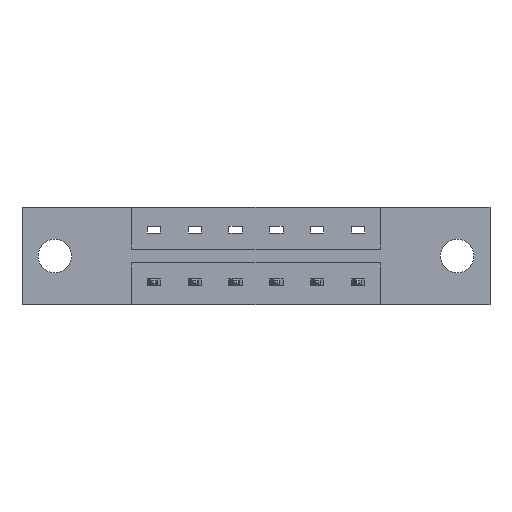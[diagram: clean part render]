
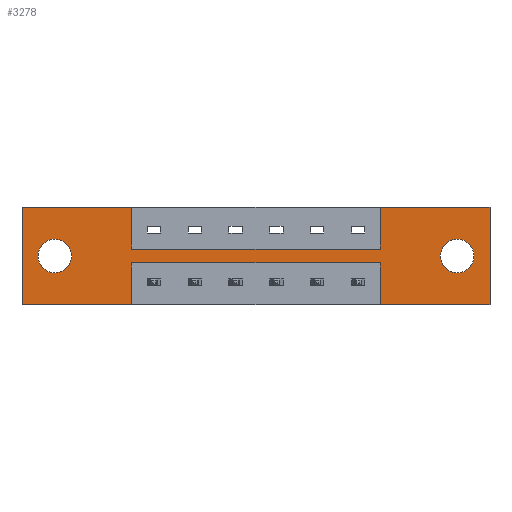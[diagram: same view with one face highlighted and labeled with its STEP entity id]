
A CAD part, front view. The second image highlights one B-rep face of the part: STEP entity #3278.
In plain terms, the highlighted planar face has unit normal (0, -1, 0).
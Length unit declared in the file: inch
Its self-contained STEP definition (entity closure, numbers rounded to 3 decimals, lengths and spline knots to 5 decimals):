
#50 = EDGE_CURVE ( 'NONE', #3558, #2212, #6643, .T. ) ;
#74 = CIRCLE ( 'NONE', #6820, 0.064 ) ;
#160 = DIRECTION ( 'NONE',  ( 0., 0., -1. ) ) ;
#168 = ORIENTED_EDGE ( 'NONE', *, *, #7767, .F. ) ;
#190 = CARTESIAN_POINT ( 'NONE',  ( 1.3665, 0., 0. ) ) ;
#343 = CARTESIAN_POINT ( 'NONE',  ( 1.784, 0., -0.37 ) ) ;
#434 = VECTOR ( 'NONE', #5804, 39.37008 ) ;
#483 = LINE ( 'NONE', #8229, #7252 ) ;
#489 = DIRECTION ( 'NONE',  ( -1., 0., 0. ) ) ;
#573 = LINE ( 'NONE', #5742, #3854 ) ;
#639 = VECTOR ( 'NONE', #5805, 39.37008 ) ;
#731 = ORIENTED_EDGE ( 'NONE', *, *, #4554, .F. ) ;
#736 = CIRCLE ( 'NONE', #7083, 0.064 ) ;
#845 = CARTESIAN_POINT ( 'NONE',  ( 0.4175, 0., -0.1585 ) ) ;
#866 = CARTESIAN_POINT ( 'NONE',  ( 0.125, 0., -0.185 ) ) ;
#899 = ORIENTED_EDGE ( 'NONE', *, *, #7003, .F. ) ;
#901 = ORIENTED_EDGE ( 'NONE', *, *, #7945, .F. ) ;
#948 = DIRECTION ( 'NONE',  ( 0., 0., -1. ) ) ;
#1079 = DIRECTION ( 'NONE',  ( -1., 0., 0. ) ) ;
#1104 = VERTEX_POINT ( 'NONE', #1747 ) ;
#1106 = CARTESIAN_POINT ( 'NONE',  ( 0., 0., -0.37 ) ) ;
#1258 = LINE ( 'NONE', #4473, #4813 ) ;
#1288 = ORIENTED_EDGE ( 'NONE', *, *, #2290, .F. ) ;
#1340 = VERTEX_POINT ( 'NONE', #7374 ) ;
#1341 = FACE_BOUND ( 'NONE', #5637, .T. ) ;
#1344 = VERTEX_POINT ( 'NONE', #4782 ) ;
#1371 = DIRECTION ( 'NONE',  ( 0., 1., 0. ) ) ;
#1386 = VERTEX_POINT ( 'NONE', #343 ) ;
#1469 = LINE ( 'NONE', #5368, #7797 ) ;
#1497 = LINE ( 'NONE', #4253, #4537 ) ;
#1504 = ORIENTED_EDGE ( 'NONE', *, *, #5845, .F. ) ;
#1539 = DIRECTION ( 'NONE',  ( 0., 0., -1. ) ) ;
#1661 = CARTESIAN_POINT ( 'NONE',  ( 1.3665, 0., -0.2115 ) ) ;
#1742 = DIRECTION ( 'NONE',  ( 0., 1., 0. ) ) ;
#1744 = ORIENTED_EDGE ( 'NONE', *, *, #50, .F. ) ;
#1747 = CARTESIAN_POINT ( 'NONE',  ( 1.659, 0., -0.121 ) ) ;
#1804 = CARTESIAN_POINT ( 'NONE',  ( 1.784, 0., 0. ) ) ;
#1864 = DIRECTION ( 'NONE',  ( -1., 0., 0. ) ) ;
#1870 = VERTEX_POINT ( 'NONE', #3134 ) ;
#1988 = VECTOR ( 'NONE', #3894, 39.37008 ) ;
#2088 = VECTOR ( 'NONE', #489, 39.37008 ) ;
#2092 = EDGE_CURVE ( 'NONE', #1340, #1344, #5871, .T. ) ;
#2192 = CARTESIAN_POINT ( 'NONE',  ( 1.659, 0., -0.249 ) ) ;
#2212 = VERTEX_POINT ( 'NONE', #6166 ) ;
#2283 = VERTEX_POINT ( 'NONE', #6288 ) ;
#2290 = EDGE_CURVE ( 'NONE', #6477, #2283, #4339, .T. ) ;
#2296 = EDGE_LOOP ( 'NONE', ( #901, #2449, #5321, #168, #4443, #1744, #6154, #899, #731, #1288, #1504, #3020 ) ) ;
#2305 = ORIENTED_EDGE ( 'NONE', *, *, #4058, .T. ) ;
#2449 = ORIENTED_EDGE ( 'NONE', *, *, #5718, .F. ) ;
#2600 = VERTEX_POINT ( 'NONE', #6654 ) ;
#2734 = ORIENTED_EDGE ( 'NONE', *, *, #2092, .T. ) ;
#2772 = VERTEX_POINT ( 'NONE', #6682 ) ;
#3020 = ORIENTED_EDGE ( 'NONE', *, *, #5200, .F. ) ;
#3050 = VECTOR ( 'NONE', #948, 39.37008 ) ;
#3134 = CARTESIAN_POINT ( 'NONE',  ( 1.3665, 0., -0.37 ) ) ;
#3217 = DIRECTION ( 'NONE',  ( 0., 0., 1. ) ) ;
#3278 = ADVANCED_FACE ( 'NONE', ( #5245, #1341, #7854 ), #3344, .T. ) ;
#3344 = PLANE ( 'NONE',  #5326 ) ;
#3387 = DIRECTION ( 'NONE',  ( 0., 1., 0. ) ) ;
#3558 = VERTEX_POINT ( 'NONE', #7043 ) ;
#3772 = DIRECTION ( 'NONE',  ( 1., 0., 0. ) ) ;
#3773 = LINE ( 'NONE', #1804, #1988 ) ;
#3792 = CARTESIAN_POINT ( 'NONE',  ( 0., 0., -0.37 ) ) ;
#3852 = AXIS2_PLACEMENT_3D ( 'NONE', #7090, #3387, #7850 ) ;
#3854 = VECTOR ( 'NONE', #3217, 39.37008 ) ;
#3860 = EDGE_CURVE ( 'NONE', #2772, #3558, #5482, .T. ) ;
#3894 = DIRECTION ( 'NONE',  ( 0., 0., -1. ) ) ;
#4058 = EDGE_CURVE ( 'NONE', #1104, #4666, #736, .T. ) ;
#4107 = ORIENTED_EDGE ( 'NONE', *, *, #7725, .T. ) ;
#4177 = CARTESIAN_POINT ( 'NONE',  ( 1.659, 0., -0.185 ) ) ;
#4253 = CARTESIAN_POINT ( 'NONE',  ( 0., 0., 0. ) ) ;
#4339 = LINE ( 'NONE', #3792, #2088 ) ;
#4369 = DIRECTION ( 'NONE',  ( 0., 0., -1. ) ) ;
#4417 = CARTESIAN_POINT ( 'NONE',  ( 0.4175, 0., -0.2115 ) ) ;
#4443 = ORIENTED_EDGE ( 'NONE', *, *, #6187, .F. ) ;
#4473 = CARTESIAN_POINT ( 'NONE',  ( 0., 0., 0. ) ) ;
#4492 = EDGE_CURVE ( 'NONE', #4607, #1386, #3773, .T. ) ;
#4537 = VECTOR ( 'NONE', #6830, 39.37008 ) ;
#4554 = EDGE_CURVE ( 'NONE', #2283, #6061, #1469, .T. ) ;
#4570 = CARTESIAN_POINT ( 'NONE',  ( 0.4175, 0., -0.2115 ) ) ;
#4607 = VERTEX_POINT ( 'NONE', #7315 ) ;
#4608 = LINE ( 'NONE', #4570, #639 ) ;
#4666 = VERTEX_POINT ( 'NONE', #2192 ) ;
#4782 = CARTESIAN_POINT ( 'NONE',  ( 0.125, 0., -0.121 ) ) ;
#4813 = VECTOR ( 'NONE', #3772, 39.37008 ) ;
#4914 = VERTEX_POINT ( 'NONE', #190 ) ;
#5200 = EDGE_CURVE ( 'NONE', #7674, #2600, #6910, .T. ) ;
#5225 = CIRCLE ( 'NONE', #7394, 0.064 ) ;
#5245 = FACE_BOUND ( 'NONE', #5327, .T. ) ;
#5316 = DIRECTION ( 'NONE',  ( 0., -1., 0. ) ) ;
#5321 = ORIENTED_EDGE ( 'NONE', *, *, #4492, .F. ) ;
#5326 = AXIS2_PLACEMENT_3D ( 'NONE', #7942, #5316, #160 ) ;
#5327 = EDGE_LOOP ( 'NONE', ( #2305, #4107 ) ) ;
#5368 = CARTESIAN_POINT ( 'NONE',  ( 0., 0., 0. ) ) ;
#5482 = LINE ( 'NONE', #6029, #3050 ) ;
#5637 = EDGE_LOOP ( 'NONE', ( #8133, #2734 ) ) ;
#5718 = EDGE_CURVE ( 'NONE', #1386, #1870, #6902, .T. ) ;
#5742 = CARTESIAN_POINT ( 'NONE',  ( 1.3665, 0., -0.1585 ) ) ;
#5804 = DIRECTION ( 'NONE',  ( 1., 0., 0. ) ) ;
#5805 = DIRECTION ( 'NONE',  ( 0., 0., -1. ) ) ;
#5845 = EDGE_CURVE ( 'NONE', #2600, #6477, #4608, .T. ) ;
#5871 = CIRCLE ( 'NONE', #3852, 0.064 ) ;
#5918 = DIRECTION ( 'NONE',  ( 0., 0., 1. ) ) ;
#6029 = CARTESIAN_POINT ( 'NONE',  ( 0.4175, 0., -0.1585 ) ) ;
#6058 = CARTESIAN_POINT ( 'NONE',  ( 0., 0., 0. ) ) ;
#6061 = VERTEX_POINT ( 'NONE', #6058 ) ;
#6154 = ORIENTED_EDGE ( 'NONE', *, *, #3860, .F. ) ;
#6166 = CARTESIAN_POINT ( 'NONE',  ( 1.3665, 0., -0.1585 ) ) ;
#6187 = EDGE_CURVE ( 'NONE', #2212, #4914, #573, .T. ) ;
#6245 = CARTESIAN_POINT ( 'NONE',  ( 0.4175, 0., -0.37 ) ) ;
#6288 = CARTESIAN_POINT ( 'NONE',  ( 0., 0., -0.37 ) ) ;
#6355 = EDGE_CURVE ( 'NONE', #1344, #1340, #74, .T. ) ;
#6477 = VERTEX_POINT ( 'NONE', #6245 ) ;
#6643 = LINE ( 'NONE', #845, #434 ) ;
#6654 = CARTESIAN_POINT ( 'NONE',  ( 0.4175, 0., -0.2115 ) ) ;
#6682 = CARTESIAN_POINT ( 'NONE',  ( 0.4175, 0., 0. ) ) ;
#6820 = AXIS2_PLACEMENT_3D ( 'NONE', #866, #1371, #7847 ) ;
#6830 = DIRECTION ( 'NONE',  ( 1., 0., 0. ) ) ;
#6902 = LINE ( 'NONE', #1106, #7411 ) ;
#6910 = LINE ( 'NONE', #4417, #7428 ) ;
#7003 = EDGE_CURVE ( 'NONE', #6061, #2772, #1258, .T. ) ;
#7043 = CARTESIAN_POINT ( 'NONE',  ( 0.4175, 0., -0.1585 ) ) ;
#7083 = AXIS2_PLACEMENT_3D ( 'NONE', #7556, #1742, #4369 ) ;
#7090 = CARTESIAN_POINT ( 'NONE',  ( 0.125, 0., -0.185 ) ) ;
#7252 = VECTOR ( 'NONE', #7633, 39.37008 ) ;
#7315 = CARTESIAN_POINT ( 'NONE',  ( 1.784, 0., 0. ) ) ;
#7374 = CARTESIAN_POINT ( 'NONE',  ( 0.125, 0., -0.249 ) ) ;
#7394 = AXIS2_PLACEMENT_3D ( 'NONE', #4177, #8144, #1539 ) ;
#7411 = VECTOR ( 'NONE', #1864, 39.37008 ) ;
#7428 = VECTOR ( 'NONE', #1079, 39.37008 ) ;
#7556 = CARTESIAN_POINT ( 'NONE',  ( 1.659, 0., -0.185 ) ) ;
#7633 = DIRECTION ( 'NONE',  ( 0., 0., 1. ) ) ;
#7674 = VERTEX_POINT ( 'NONE', #1661 ) ;
#7725 = EDGE_CURVE ( 'NONE', #4666, #1104, #5225, .T. ) ;
#7767 = EDGE_CURVE ( 'NONE', #4914, #4607, #1497, .T. ) ;
#7797 = VECTOR ( 'NONE', #5918, 39.37008 ) ;
#7847 = DIRECTION ( 'NONE',  ( 0., 0., 1. ) ) ;
#7850 = DIRECTION ( 'NONE',  ( 0., 0., 1. ) ) ;
#7854 = FACE_OUTER_BOUND ( 'NONE', #2296, .T. ) ;
#7942 = CARTESIAN_POINT ( 'NONE',  ( 0., 0., -0.37 ) ) ;
#7945 = EDGE_CURVE ( 'NONE', #1870, #7674, #483, .T. ) ;
#8133 = ORIENTED_EDGE ( 'NONE', *, *, #6355, .T. ) ;
#8144 = DIRECTION ( 'NONE',  ( 0., 1., 0. ) ) ;
#8229 = CARTESIAN_POINT ( 'NONE',  ( 1.3665, 0., -0.2115 ) ) ;
